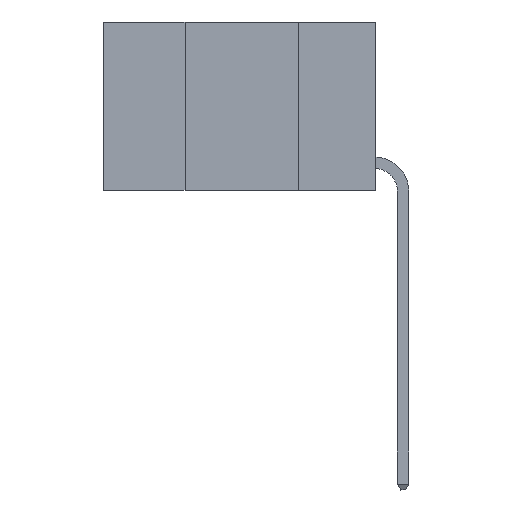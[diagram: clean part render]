
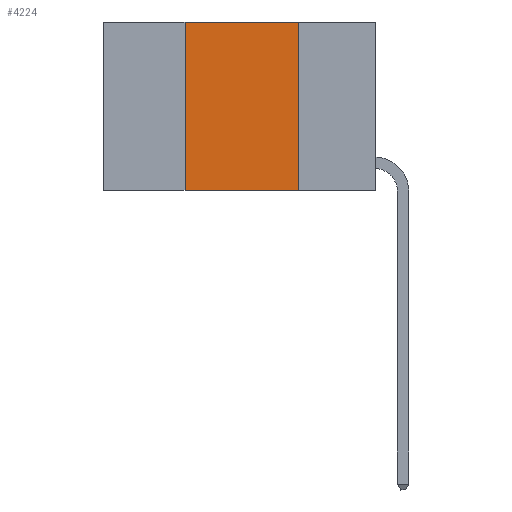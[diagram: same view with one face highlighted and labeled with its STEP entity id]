
A CAD part, left-side view. The second image highlights one B-rep face of the part: STEP entity #4224.
In plain terms, the highlighted planar face has unit normal (-1, 0, 0).
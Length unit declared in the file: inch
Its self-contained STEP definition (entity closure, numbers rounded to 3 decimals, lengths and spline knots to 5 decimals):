
#3145 = CARTESIAN_POINT ( 'NONE',  ( 0., 0.42, 0. ) ) ;
#3305 = DIRECTION ( 'NONE',  ( 0., 0., -1. ) ) ;
#4224 = ADVANCED_FACE ( 'NONE', ( #18434 ), #6268, .F. ) ;
#4435 = LINE ( 'NONE', #3145, #13934 ) ;
#5815 = ORIENTED_EDGE ( 'NONE', *, *, #12802, .F. ) ;
#6202 = VERTEX_POINT ( 'NONE', #12558 ) ;
#6268 = PLANE ( 'NONE',  #7923 ) ;
#6429 = ORIENTED_EDGE ( 'NONE', *, *, #15533, .F. ) ;
#6783 = VECTOR ( 'NONE', #7524, 39.37008 ) ;
#7394 = LINE ( 'NONE', #14846, #14989 ) ;
#7524 = DIRECTION ( 'NONE',  ( 0., -1., 0. ) ) ;
#7876 = EDGE_CURVE ( 'NONE', #8237, #11383, #4435, .T. ) ;
#7877 = DIRECTION ( 'NONE',  ( 0., 0., 1. ) ) ;
#7923 = AXIS2_PLACEMENT_3D ( 'NONE', #9101, #16956, #3305 ) ;
#8005 = CARTESIAN_POINT ( 'NONE',  ( 0., 0.17, -0.37 ) ) ;
#8110 = VECTOR ( 'NONE', #9862, 39.37008 ) ;
#8237 = VERTEX_POINT ( 'NONE', #11778 ) ;
#8241 = CARTESIAN_POINT ( 'NONE',  ( 0., 0.42, 0. ) ) ;
#8764 = VERTEX_POINT ( 'NONE', #8005 ) ;
#9101 = CARTESIAN_POINT ( 'NONE',  ( 0., 0.6, 0. ) ) ;
#9105 = EDGE_CURVE ( 'NONE', #8237, #8764, #7394, .T. ) ;
#9862 = DIRECTION ( 'NONE',  ( 0., 0., -1. ) ) ;
#11383 = VERTEX_POINT ( 'NONE', #8241 ) ;
#11778 = CARTESIAN_POINT ( 'NONE',  ( 0., 0.42, -0.37 ) ) ;
#11843 = LINE ( 'NONE', #16553, #6783 ) ;
#12558 = CARTESIAN_POINT ( 'NONE',  ( 0., 0.17, 0. ) ) ;
#12802 = EDGE_CURVE ( 'NONE', #11383, #6202, #11843, .T. ) ;
#12811 = CARTESIAN_POINT ( 'NONE',  ( 0., 0.17, 0. ) ) ;
#13456 = EDGE_LOOP ( 'NONE', ( #6429, #5815, #15694, #16203 ) ) ;
#13934 = VECTOR ( 'NONE', #7877, 39.37008 ) ;
#14179 = LINE ( 'NONE', #12811, #8110 ) ;
#14846 = CARTESIAN_POINT ( 'NONE',  ( 0., 0.6, -0.37 ) ) ;
#14989 = VECTOR ( 'NONE', #16139, 39.37008 ) ;
#15533 = EDGE_CURVE ( 'NONE', #6202, #8764, #14179, .T. ) ;
#15694 = ORIENTED_EDGE ( 'NONE', *, *, #7876, .F. ) ;
#16139 = DIRECTION ( 'NONE',  ( 0., -1., 0. ) ) ;
#16203 = ORIENTED_EDGE ( 'NONE', *, *, #9105, .T. ) ;
#16553 = CARTESIAN_POINT ( 'NONE',  ( 0., 0.6, 0. ) ) ;
#16956 = DIRECTION ( 'NONE',  ( 1., 0., 0. ) ) ;
#18434 = FACE_OUTER_BOUND ( 'NONE', #13456, .T. ) ;
